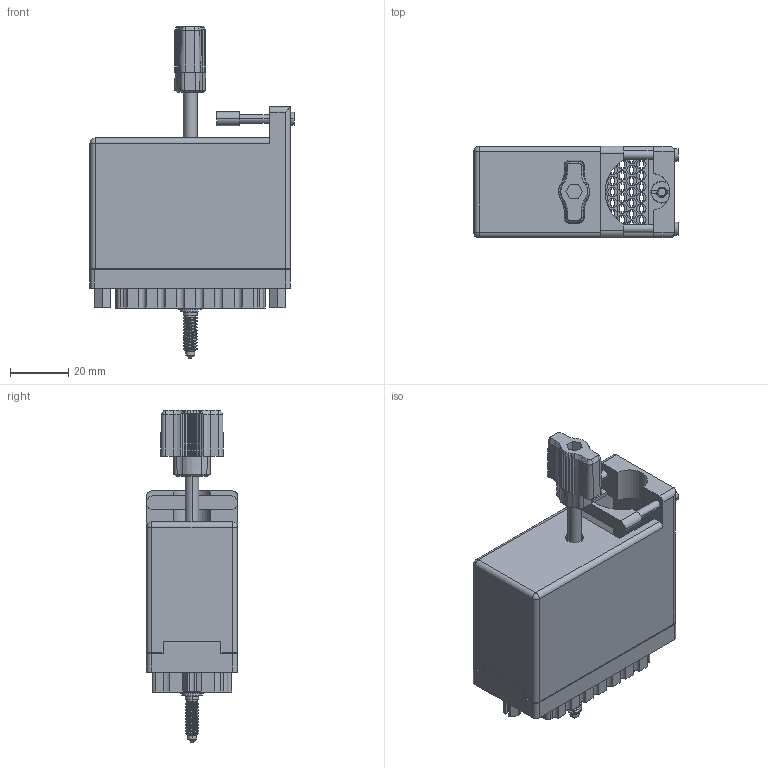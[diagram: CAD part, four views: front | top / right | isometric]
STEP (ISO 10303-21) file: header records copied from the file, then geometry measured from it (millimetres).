
FILE_DESCRIPTION (( 'STEP AP203' ), '1' );
FILE_NAME ('516-090-000-661.STEP', '2020-03-06T17:03:31', ( '' ), ( '' ), 'SwSTEP 2.0', 'SolidWorks 2016', '' );
FILE_SCHEMA (( 'CONFIG_CONTROL_DESIGN' ));
Length unit declared in the file: inch
Products named in the file (13): 516-250-091-111; 516 Part Receptacle_090; 516-253-095-100; 516-230-001_Metal - 090 Top Entry; 516-221-090-102_091; Actuating Screw Assy 090-120; 516-252-091-102; Grub Screw; 516-090-000-661; 516-251-095-100; 516-253-190-107; 516-254-091-109; 516-221-090-102_090
Assembly tree (14 placements, depth 3):
  516-090-000-661
    516 Part Receptacle_090
    516-230-001_Metal - 090 Top Entry
    516-252-091-102  x2
    516-221-090-102_090
    Actuating Screw Assy 090-120
      516-251-095-100
      516-254-091-109
      516-253-095-100  x2
      516-253-190-107
      516-250-091-111
      Grub Screw
    516-221-090-102_091
Bounding box: 70.31 x 31.34 x 114.34 mm (x, y, z)
Volume: 40583.3 mm3; surface area: 57382.7 mm2
Topology: 13 solids, 13 shells, 2446 faces, 7073 edges, 4672 vertices
Faces by surface type: plane 1566, cylinder 743, cone 96, bspline 39, sphere 2
Entity records: 93136 total; most frequent: CARTESIAN_POINT 26923, ORIENTED_EDGE 13954, DIRECTION 13237, EDGE_CURVE 6977, VECTOR 4803, LINE 4803, VERTEX_POINT 4612, AXIS2_PLACEMENT_3D 4217
